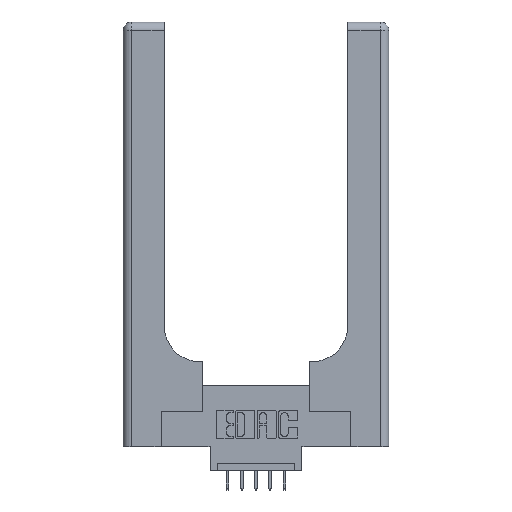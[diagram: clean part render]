
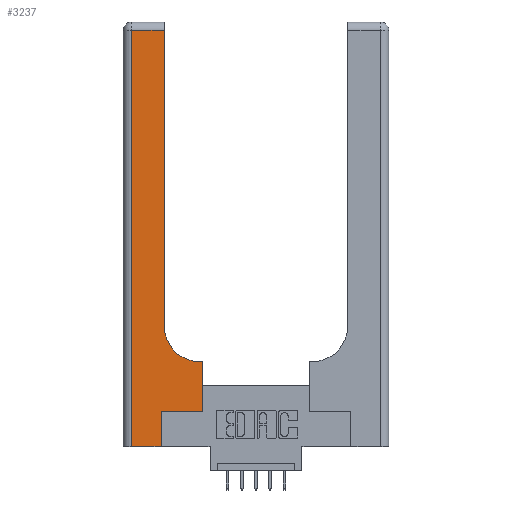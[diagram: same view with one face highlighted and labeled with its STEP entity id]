
A CAD part, top view. The second image highlights one B-rep face of the part: STEP entity #3237.
In plain terms, the highlighted planar face has unit normal (0, 0, 1).
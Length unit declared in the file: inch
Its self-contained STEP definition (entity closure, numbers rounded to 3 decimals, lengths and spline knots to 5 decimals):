
#21 = VECTOR ( 'NONE', #12713, 39.37008 ) ;
#215 = CARTESIAN_POINT ( 'NONE',  ( 0.269, 0.25, 0.37 ) ) ;
#249 = DIRECTION ( 'NONE',  ( 0., 1., 0. ) ) ;
#332 = CARTESIAN_POINT ( 'NONE',  ( 0.2915, 3., 0.37 ) ) ;
#437 = FACE_OUTER_BOUND ( 'NONE', #11492, .T. ) ;
#690 = VERTEX_POINT ( 'NONE', #7998 ) ;
#783 = CARTESIAN_POINT ( 'NONE',  ( 0.269, 0., 0.37 ) ) ;
#1079 = VECTOR ( 'NONE', #11288, 39.37008 ) ;
#1222 = VERTEX_POINT ( 'NONE', #6445 ) ;
#1326 = CARTESIAN_POINT ( 'NONE',  ( 0.2915, 0.6, 0.37 ) ) ;
#1328 = AXIS2_PLACEMENT_3D ( 'NONE', #13623, #13552, #3827 ) ;
#1332 = VERTEX_POINT ( 'NONE', #9699 ) ;
#1605 = DIRECTION ( 'NONE',  ( -1., 0., 0. ) ) ;
#1667 = EDGE_CURVE ( 'NONE', #12960, #1332, #11194, .T. ) ;
#1671 = EDGE_CURVE ( 'NONE', #6481, #690, #7669, .T. ) ;
#1700 = ORIENTED_EDGE ( 'NONE', *, *, #1671, .T. ) ;
#1911 = EDGE_CURVE ( 'NONE', #2181, #1222, #10378, .T. ) ;
#2181 = VERTEX_POINT ( 'NONE', #9167 ) ;
#2626 = LINE ( 'NONE', #332, #8667 ) ;
#2706 = VECTOR ( 'NONE', #13350, 39.37008 ) ;
#2804 = CARTESIAN_POINT ( 'NONE',  ( 0., 3., 0.37 ) ) ;
#2974 = CARTESIAN_POINT ( 'NONE',  ( 0.06, 0., 0.37 ) ) ;
#3194 = LINE ( 'NONE', #7545, #7309 ) ;
#3237 = ADVANCED_FACE ( 'NONE', ( #437 ), #13671, .F. ) ;
#3329 = DIRECTION ( 'NONE',  ( 0., 1., 0. ) ) ;
#3465 = ORIENTED_EDGE ( 'NONE', *, *, #1911, .T. ) ;
#3711 = EDGE_CURVE ( 'NONE', #7566, #6481, #7414, .T. ) ;
#3827 = DIRECTION ( 'NONE',  ( 1., 0., 0. ) ) ;
#3870 = DIRECTION ( 'NONE',  ( 0., 0., -1. ) ) ;
#3980 = CARTESIAN_POINT ( 'NONE',  ( 0.5585, 0.6, 0.37 ) ) ;
#4496 = ORIENTED_EDGE ( 'NONE', *, *, #10360, .T. ) ;
#4670 = CARTESIAN_POINT ( 'NONE',  ( 0.269, 0., 0.37 ) ) ;
#4687 = LINE ( 'NONE', #13419, #2706 ) ;
#4732 = ORIENTED_EDGE ( 'NONE', *, *, #3711, .T. ) ;
#5058 = CARTESIAN_POINT ( 'NONE',  ( 0., 0., 0.37 ) ) ;
#5761 = ORIENTED_EDGE ( 'NONE', *, *, #6792, .T. ) ;
#5882 = CIRCLE ( 'NONE', #1328, 0.25 ) ;
#6041 = ORIENTED_EDGE ( 'NONE', *, *, #1667, .T. ) ;
#6093 = VECTOR ( 'NONE', #6680, 39.37008 ) ;
#6445 = CARTESIAN_POINT ( 'NONE',  ( 0.06, 2.94, 0.37 ) ) ;
#6481 = VERTEX_POINT ( 'NONE', #783 ) ;
#6680 = DIRECTION ( 'NONE',  ( -1., 0., 0. ) ) ;
#6792 = EDGE_CURVE ( 'NONE', #690, #7490, #11013, .T. ) ;
#6886 = DIRECTION ( 'NONE',  ( -1., 0., 0. ) ) ;
#6962 = CARTESIAN_POINT ( 'NONE',  ( 0.2915, 0.85, 0.37 ) ) ;
#7309 = VECTOR ( 'NONE', #3329, 39.37008 ) ;
#7414 = LINE ( 'NONE', #5058, #21 ) ;
#7437 = EDGE_CURVE ( 'NONE', #1332, #9011, #5882, .T. ) ;
#7490 = VERTEX_POINT ( 'NONE', #8532 ) ;
#7538 = ORIENTED_EDGE ( 'NONE', *, *, #10073, .T. ) ;
#7545 = CARTESIAN_POINT ( 'NONE',  ( 0.5585, 0.25, 0.37 ) ) ;
#7566 = VERTEX_POINT ( 'NONE', #2974 ) ;
#7669 = LINE ( 'NONE', #4670, #10437 ) ;
#7998 = CARTESIAN_POINT ( 'NONE',  ( 0.269, 0.25, 0.37 ) ) ;
#8505 = EDGE_CURVE ( 'NONE', #1222, #7566, #4687, .T. ) ;
#8532 = CARTESIAN_POINT ( 'NONE',  ( 0.5585, 0.25, 0.37 ) ) ;
#8667 = VECTOR ( 'NONE', #12219, 39.37008 ) ;
#9011 = VERTEX_POINT ( 'NONE', #6962 ) ;
#9167 = CARTESIAN_POINT ( 'NONE',  ( 0.2915, 2.94, 0.37 ) ) ;
#9599 = AXIS2_PLACEMENT_3D ( 'NONE', #2804, #3870, #6886 ) ;
#9699 = CARTESIAN_POINT ( 'NONE',  ( 0.5415, 0.6, 0.37 ) ) ;
#10073 = EDGE_CURVE ( 'NONE', #9011, #2181, #2626, .T. ) ;
#10360 = EDGE_CURVE ( 'NONE', #7490, #12960, #3194, .T. ) ;
#10378 = LINE ( 'NONE', #11393, #13183 ) ;
#10437 = VECTOR ( 'NONE', #249, 39.37008 ) ;
#11013 = LINE ( 'NONE', #215, #1079 ) ;
#11194 = LINE ( 'NONE', #1326, #6093 ) ;
#11288 = DIRECTION ( 'NONE',  ( 1., 0., 0. ) ) ;
#11393 = CARTESIAN_POINT ( 'NONE',  ( 0., 2.94, 0.37 ) ) ;
#11492 = EDGE_LOOP ( 'NONE', ( #7538, #3465, #12370, #4732, #1700, #5761, #4496, #6041, #12836 ) ) ;
#12219 = DIRECTION ( 'NONE',  ( 0., 1., 0. ) ) ;
#12370 = ORIENTED_EDGE ( 'NONE', *, *, #8505, .T. ) ;
#12713 = DIRECTION ( 'NONE',  ( 1., 0., 0. ) ) ;
#12836 = ORIENTED_EDGE ( 'NONE', *, *, #7437, .T. ) ;
#12960 = VERTEX_POINT ( 'NONE', #3980 ) ;
#13183 = VECTOR ( 'NONE', #1605, 39.37008 ) ;
#13350 = DIRECTION ( 'NONE',  ( 0., -1., 0. ) ) ;
#13419 = CARTESIAN_POINT ( 'NONE',  ( 0.06, 3., 0.37 ) ) ;
#13552 = DIRECTION ( 'NONE',  ( 0., 0., -1. ) ) ;
#13623 = CARTESIAN_POINT ( 'NONE',  ( 0.5415, 0.85, 0.37 ) ) ;
#13671 = PLANE ( 'NONE',  #9599 ) ;
